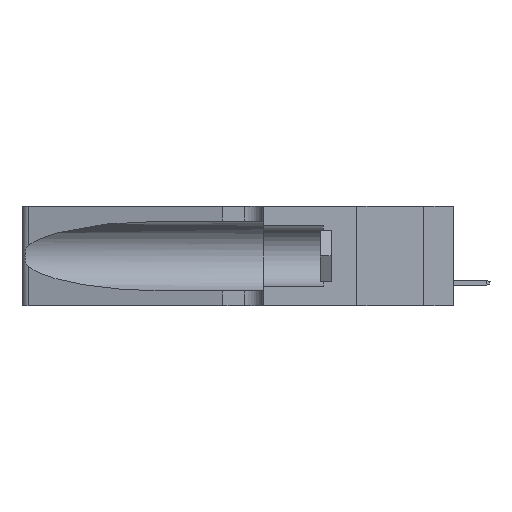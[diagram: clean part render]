
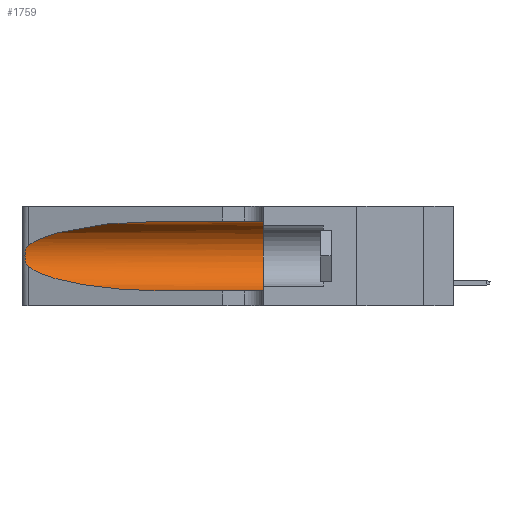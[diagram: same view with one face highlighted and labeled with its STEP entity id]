
A CAD part, left-side view. The second image highlights one B-rep face of the part: STEP entity #1759.
In plain terms, the highlighted cylindrical face has radius 3.308 mm (diameter 6.617 mm), a partial arc.
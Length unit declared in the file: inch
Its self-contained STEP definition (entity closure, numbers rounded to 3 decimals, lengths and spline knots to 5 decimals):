
#620 = CARTESIAN_POINT ( 'NONE',  ( 0.26018, 1.23835, 0.19895 ) ) ;
#1125 = CARTESIAN_POINT ( 'NONE',  ( 0.25487, 1.22718, 0.14631 ) ) ;
#1759 = ADVANCED_FACE ( 'NONE', ( #21779 ), #33037, .F. ) ;
#2546 = DIRECTION ( 'NONE',  ( 0., -1., 0. ) ) ;
#4940 =( BOUNDED_CURVE ( )  B_SPLINE_CURVE ( 3, ( #38339, #45864, #26328, #49105 ),
 .UNSPECIFIED., .F., .T. ) 
 B_SPLINE_CURVE_WITH_KNOTS ( ( 4, 4 ),
 ( 1.5708, 2.84003 ),
 .UNSPECIFIED. ) 
 CURVE ( )  GEOMETRIC_REPRESENTATION_ITEM ( )  RATIONAL_B_SPLINE_CURVE ( ( 1., 0.87, 0.87, 1. ) ) 
 REPRESENTATION_ITEM ( '' )  );
#6111 = CARTESIAN_POINT ( 'NONE',  ( 0.1305, 0.72297, 0.31525 ) ) ;
#8346 = CARTESIAN_POINT ( 'NONE',  ( 0.1305, 1.61858, 0.05475 ) ) ;
#9826 = B_SPLINE_CURVE_WITH_KNOTS ( 'NONE', 3,
 ( #16112, #23105, #31609, #38652, #20107, #620, #38392, #19356, #38902, #34604, #35372, #46935, #35113, #1125 ),
 .UNSPECIFIED., .F., .F.,
 ( 4, 2, 2, 2, 2, 2, 4 ),
 ( 0., 0.00027, 0.00053, 0.00107, 0.0016, 0.00187, 0.00214 ),
 .UNSPECIFIED. ) ;
#11074 = ORIENTED_EDGE ( 'NONE', *, *, #15023, .T. ) ;
#13107 = VECTOR ( 'NONE', #22131, 39.37008 ) ;
#13422 = VERTEX_POINT ( 'NONE', #6111 ) ;
#15023 = EDGE_CURVE ( 'NONE', #19880, #38104, #48764, .T. ) ;
#15400 = ORIENTED_EDGE ( 'NONE', *, *, #48510, .T. ) ;
#15843 = DIRECTION ( 'NONE',  ( 0., -1., 0. ) ) ;
#15913 = AXIS2_PLACEMENT_3D ( 'NONE', #44591, #2546, #36560 ) ;
#16112 = CARTESIAN_POINT ( 'NONE',  ( 0.25487, 1.22718, 0.22369 ) ) ;
#18398 = CARTESIAN_POINT ( 'NONE',  ( 0.1305, 1.61858, 0.31525 ) ) ;
#18886 = LINE ( 'NONE', #18398, #13107 ) ;
#19356 = CARTESIAN_POINT ( 'NONE',  ( 0.26075, 1.23896, 0.178 ) ) ;
#19880 = VERTEX_POINT ( 'NONE', #24948 ) ;
#20107 = CARTESIAN_POINT ( 'NONE',  ( 0.25854, 1.2359, 0.20912 ) ) ;
#21314 = CARTESIAN_POINT ( 'NONE',  ( 0.1305, 0.72297, 0.05475 ) ) ;
#21779 = FACE_OUTER_BOUND ( 'NONE', #25888, .T. ) ;
#22131 = DIRECTION ( 'NONE',  ( 0., -1., 0. ) ) ;
#22761 = CARTESIAN_POINT ( 'NONE',  ( 0.1305, 0.35, 0.31525 ) ) ;
#23036 = ORIENTED_EDGE ( 'NONE', *, *, #39841, .T. ) ;
#23105 = CARTESIAN_POINT ( 'NONE',  ( 0.25555, 1.22994, 0.2215 ) ) ;
#23126 = EDGE_CURVE ( 'NONE', #13422, #28470, #18886, .T. ) ;
#24863 = EDGE_CURVE ( 'NONE', #28470, #44833, #46020, .T. ) ;
#24948 = CARTESIAN_POINT ( 'NONE',  ( 0.25487, 1.22718, 0.14631 ) ) ;
#25888 = EDGE_LOOP ( 'NONE', ( #33332, #23036, #11074, #15400, #31074, #36336 ) ) ;
#26328 = CARTESIAN_POINT ( 'NONE',  ( 0.2373, 1.15595, 0.28018 ) ) ;
#28452 = AXIS2_PLACEMENT_3D ( 'NONE', #37361, #48876, #30097 ) ;
#28470 = VERTEX_POINT ( 'NONE', #22761 ) ;
#30097 = DIRECTION ( 'NONE',  ( 0., 0., 1. ) ) ;
#31074 = ORIENTED_EDGE ( 'NONE', *, *, #24863, .F. ) ;
#31609 = CARTESIAN_POINT ( 'NONE',  ( 0.25639, 1.23184, 0.21858 ) ) ;
#32103 = CARTESIAN_POINT ( 'NONE',  ( 0.18966, 0.96281, 0.05475 ) ) ;
#32340 = CARTESIAN_POINT ( 'NONE',  ( 0.25487, 1.22718, 0.14631 ) ) ;
#33037 = CYLINDRICAL_SURFACE ( 'NONE', #15913, 0.13025 ) ;
#33332 = ORIENTED_EDGE ( 'NONE', *, *, #36396, .T. ) ;
#34299 = CARTESIAN_POINT ( 'NONE',  ( 0.1305, 0.35, 0.05475 ) ) ;
#34604 = CARTESIAN_POINT ( 'NONE',  ( 0.25856, 1.23593, 0.16098 ) ) ;
#34664 = CARTESIAN_POINT ( 'NONE',  ( 0.1305, 0.72297, 0.05475 ) ) ;
#35113 = CARTESIAN_POINT ( 'NONE',  ( 0.25555, 1.22993, 0.14849 ) ) ;
#35372 = CARTESIAN_POINT ( 'NONE',  ( 0.25789, 1.23486, 0.15765 ) ) ;
#36121 = CARTESIAN_POINT ( 'NONE',  ( 0.2373, 1.15595, 0.08982 ) ) ;
#36336 = ORIENTED_EDGE ( 'NONE', *, *, #23126, .F. ) ;
#36396 = EDGE_CURVE ( 'NONE', #13422, #49160, #4940, .T. ) ;
#36527 = CARTESIAN_POINT ( 'NONE',  ( 0.25487, 1.22718, 0.22369 ) ) ;
#36560 = DIRECTION ( 'NONE',  ( 0., 0., -1. ) ) ;
#37361 = CARTESIAN_POINT ( 'NONE',  ( 0.1305, 0.35, 0.185 ) ) ;
#37669 = VECTOR ( 'NONE', #15843, 39.37008 ) ;
#38104 = VERTEX_POINT ( 'NONE', #34664 ) ;
#38339 = CARTESIAN_POINT ( 'NONE',  ( 0.1305, 0.72297, 0.31525 ) ) ;
#38392 = CARTESIAN_POINT ( 'NONE',  ( 0.26075, 1.23896, 0.19203 ) ) ;
#38652 = CARTESIAN_POINT ( 'NONE',  ( 0.25787, 1.23484, 0.2124 ) ) ;
#38902 = CARTESIAN_POINT ( 'NONE',  ( 0.26017, 1.23833, 0.17102 ) ) ;
#39159 = LINE ( 'NONE', #8346, #37669 ) ;
#39841 = EDGE_CURVE ( 'NONE', #49160, #19880, #9826, .T. ) ;
#44591 = CARTESIAN_POINT ( 'NONE',  ( 0.1305, 1.61858, 0.185 ) ) ;
#44833 = VERTEX_POINT ( 'NONE', #34299 ) ;
#45864 = CARTESIAN_POINT ( 'NONE',  ( 0.18966, 0.96281, 0.31525 ) ) ;
#46020 = CIRCLE ( 'NONE', #28452, 0.13025 ) ;
#46935 = CARTESIAN_POINT ( 'NONE',  ( 0.25639, 1.23186, 0.15144 ) ) ;
#48510 = EDGE_CURVE ( 'NONE', #38104, #44833, #39159, .T. ) ;
#48764 =( BOUNDED_CURVE ( )  B_SPLINE_CURVE ( 3, ( #32340, #36121, #32103, #21314 ),
 .UNSPECIFIED., .F., .T. ) 
 B_SPLINE_CURVE_WITH_KNOTS ( ( 4, 4 ),
 ( 3.44316, 4.71239 ),
 .UNSPECIFIED. ) 
 CURVE ( )  GEOMETRIC_REPRESENTATION_ITEM ( )  RATIONAL_B_SPLINE_CURVE ( ( 1., 0.87, 0.87, 1. ) ) 
 REPRESENTATION_ITEM ( '' )  );
#48876 = DIRECTION ( 'NONE',  ( 0., 1., 0. ) ) ;
#49105 = CARTESIAN_POINT ( 'NONE',  ( 0.25487, 1.22718, 0.22369 ) ) ;
#49160 = VERTEX_POINT ( 'NONE', #36527 ) ;
